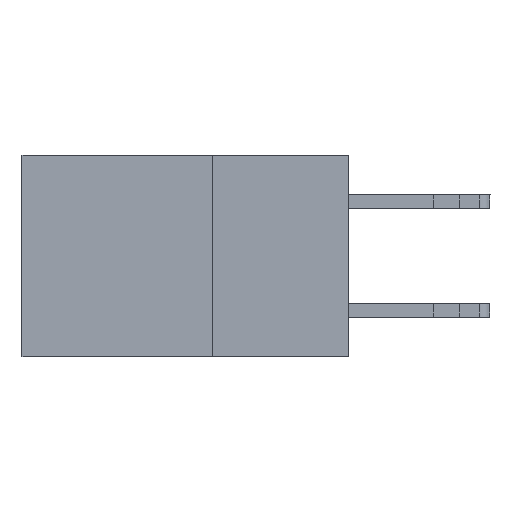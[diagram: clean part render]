
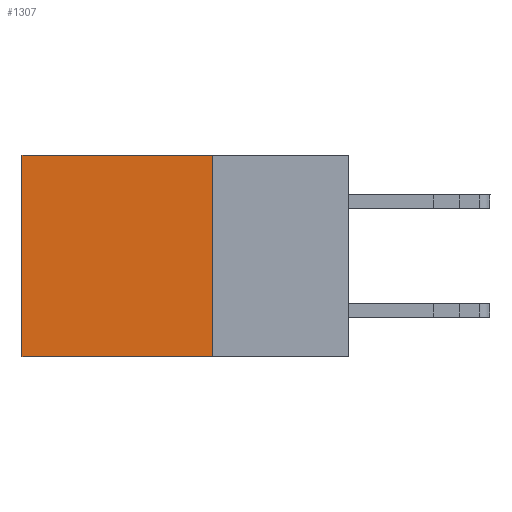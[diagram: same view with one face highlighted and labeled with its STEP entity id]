
A CAD part, left-side view. The second image highlights one B-rep face of the part: STEP entity #1307.
In plain terms, the highlighted planar face has unit normal (-1, 0, 0).
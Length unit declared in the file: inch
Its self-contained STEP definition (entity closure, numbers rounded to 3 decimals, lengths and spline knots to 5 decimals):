
#292 = LINE ( 'NONE', #3562, #7156 ) ;
#371 = VECTOR ( 'NONE', #14080, 39.37008 ) ;
#835 = CARTESIAN_POINT ( 'NONE',  ( 0.298, 0.25, -0.37 ) ) ;
#1249 = CARTESIAN_POINT ( 'NONE',  ( 0.298, 0.6, -0.37 ) ) ;
#1307 = ADVANCED_FACE ( 'NONE', ( #3822 ), #9383, .F. ) ;
#1998 = VERTEX_POINT ( 'NONE', #1249 ) ;
#2407 = EDGE_CURVE ( 'NONE', #8313, #9271, #12556, .T. ) ;
#2514 = VERTEX_POINT ( 'NONE', #835 ) ;
#2863 = LINE ( 'NONE', #8431, #9076 ) ;
#3562 = CARTESIAN_POINT ( 'NONE',  ( 0.298, 0.6, 0. ) ) ;
#3822 = FACE_OUTER_BOUND ( 'NONE', #12895, .T. ) ;
#5969 = ORIENTED_EDGE ( 'NONE', *, *, #2407, .T. ) ;
#6581 = ORIENTED_EDGE ( 'NONE', *, *, #14672, .F. ) ;
#6775 = AXIS2_PLACEMENT_3D ( 'NONE', #8221, #16667, #16762 ) ;
#7156 = VECTOR ( 'NONE', #12191, 39.37008 ) ;
#7293 = ORIENTED_EDGE ( 'NONE', *, *, #15524, .F. ) ;
#8221 = CARTESIAN_POINT ( 'NONE',  ( 0.298, 0.25, 0. ) ) ;
#8313 = VERTEX_POINT ( 'NONE', #14808 ) ;
#8431 = CARTESIAN_POINT ( 'NONE',  ( 0.298, 0.25, -0.37 ) ) ;
#8515 = CARTESIAN_POINT ( 'NONE',  ( 0.298, 0.25, 0. ) ) ;
#9076 = VECTOR ( 'NONE', #13029, 39.37008 ) ;
#9271 = VERTEX_POINT ( 'NONE', #13304 ) ;
#9383 = PLANE ( 'NONE',  #6775 ) ;
#9934 = LINE ( 'NONE', #18735, #13025 ) ;
#12063 = ORIENTED_EDGE ( 'NONE', *, *, #13507, .T. ) ;
#12191 = DIRECTION ( 'NONE',  ( 0., 0., -1. ) ) ;
#12556 = LINE ( 'NONE', #8515, #371 ) ;
#12895 = EDGE_LOOP ( 'NONE', ( #12063, #7293, #6581, #5969 ) ) ;
#13025 = VECTOR ( 'NONE', #15865, 39.37008 ) ;
#13029 = DIRECTION ( 'NONE',  ( 0., 1., 0. ) ) ;
#13304 = CARTESIAN_POINT ( 'NONE',  ( 0.298, 0.6, 0. ) ) ;
#13507 = EDGE_CURVE ( 'NONE', #9271, #1998, #292, .T. ) ;
#14080 = DIRECTION ( 'NONE',  ( 0., 1., 0. ) ) ;
#14672 = EDGE_CURVE ( 'NONE', #8313, #2514, #9934, .T. ) ;
#14808 = CARTESIAN_POINT ( 'NONE',  ( 0.298, 0.25, 0. ) ) ;
#15524 = EDGE_CURVE ( 'NONE', #2514, #1998, #2863, .T. ) ;
#15865 = DIRECTION ( 'NONE',  ( 0., 0., -1. ) ) ;
#16667 = DIRECTION ( 'NONE',  ( 1., 0., 0. ) ) ;
#16762 = DIRECTION ( 'NONE',  ( 0., 0., -1. ) ) ;
#18735 = CARTESIAN_POINT ( 'NONE',  ( 0.298, 0.25, 0. ) ) ;
